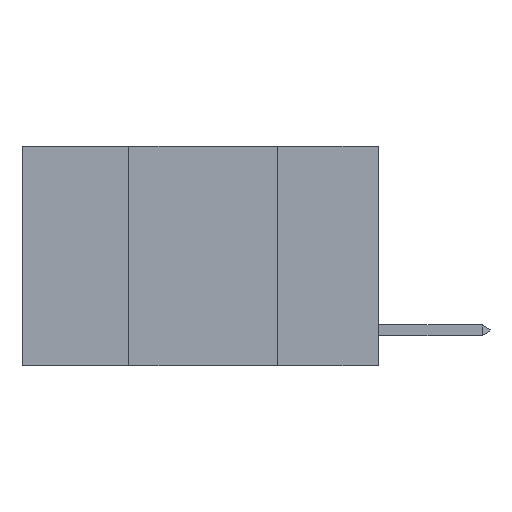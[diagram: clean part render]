
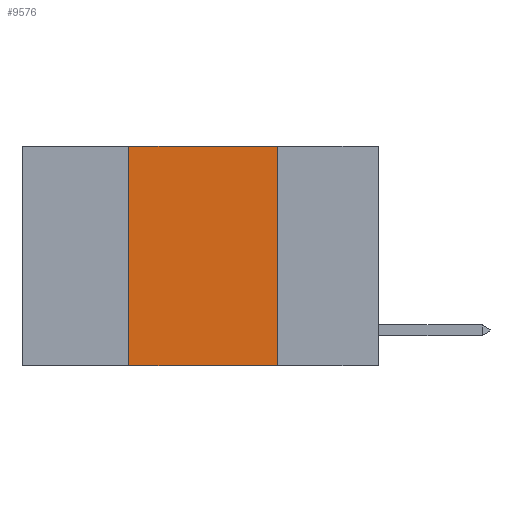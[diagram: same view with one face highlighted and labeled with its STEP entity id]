
A CAD part, left-side view. The second image highlights one B-rep face of the part: STEP entity #9576.
In plain terms, the highlighted planar face has unit normal (-1, 0, 0).
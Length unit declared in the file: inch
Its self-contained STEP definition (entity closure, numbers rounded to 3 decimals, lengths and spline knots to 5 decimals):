
#355 = VERTEX_POINT ( 'NONE', #8555 ) ;
#1116 = EDGE_CURVE ( 'NONE', #13549, #15274, #14706, .T. ) ;
#1256 = VECTOR ( 'NONE', #15183, 39.37008 ) ;
#1511 = CARTESIAN_POINT ( 'NONE',  ( 0., 0.6, 0. ) ) ;
#2590 = CARTESIAN_POINT ( 'NONE',  ( 0., 0.42, -0.37 ) ) ;
#3362 = ORIENTED_EDGE ( 'NONE', *, *, #14846, .T. ) ;
#4277 = PLANE ( 'NONE',  #7768 ) ;
#4465 = DIRECTION ( 'NONE',  ( 0., 0., -1. ) ) ;
#5555 = FACE_OUTER_BOUND ( 'NONE', #8623, .T. ) ;
#7768 = AXIS2_PLACEMENT_3D ( 'NONE', #18948, #8563, #4465 ) ;
#8332 = EDGE_CURVE ( 'NONE', #15429, #355, #17656, .T. ) ;
#8555 = CARTESIAN_POINT ( 'NONE',  ( 0., 0.42, 0. ) ) ;
#8563 = DIRECTION ( 'NONE',  ( 1., 0., 0. ) ) ;
#8623 = EDGE_LOOP ( 'NONE', ( #14347, #12231, #17965, #3362 ) ) ;
#8728 = CARTESIAN_POINT ( 'NONE',  ( 0., 0.17, 0. ) ) ;
#8741 = DIRECTION ( 'NONE',  ( 0., 0., 1. ) ) ;
#8814 = DIRECTION ( 'NONE',  ( 0., 0., -1. ) ) ;
#9192 = LINE ( 'NONE', #19212, #1256 ) ;
#9576 = ADVANCED_FACE ( 'NONE', ( #5555 ), #4277, .F. ) ;
#11822 = VECTOR ( 'NONE', #8814, 39.37008 ) ;
#12027 = DIRECTION ( 'NONE',  ( 0., -1., 0. ) ) ;
#12231 = ORIENTED_EDGE ( 'NONE', *, *, #13913, .F. ) ;
#13229 = LINE ( 'NONE', #1511, #17249 ) ;
#13549 = VERTEX_POINT ( 'NONE', #8728 ) ;
#13913 = EDGE_CURVE ( 'NONE', #355, #13549, #13229, .T. ) ;
#14347 = ORIENTED_EDGE ( 'NONE', *, *, #1116, .F. ) ;
#14706 = LINE ( 'NONE', #16447, #11822 ) ;
#14846 = EDGE_CURVE ( 'NONE', #15429, #15274, #9192, .T. ) ;
#15183 = DIRECTION ( 'NONE',  ( 0., -1., 0. ) ) ;
#15274 = VERTEX_POINT ( 'NONE', #17601 ) ;
#15429 = VERTEX_POINT ( 'NONE', #2590 ) ;
#16447 = CARTESIAN_POINT ( 'NONE',  ( 0., 0.17, 0. ) ) ;
#17249 = VECTOR ( 'NONE', #12027, 39.37008 ) ;
#17601 = CARTESIAN_POINT ( 'NONE',  ( 0., 0.17, -0.37 ) ) ;
#17656 = LINE ( 'NONE', #19035, #18620 ) ;
#17965 = ORIENTED_EDGE ( 'NONE', *, *, #8332, .F. ) ;
#18620 = VECTOR ( 'NONE', #8741, 39.37008 ) ;
#18948 = CARTESIAN_POINT ( 'NONE',  ( 0., 0.6, 0. ) ) ;
#19035 = CARTESIAN_POINT ( 'NONE',  ( 0., 0.42, 0. ) ) ;
#19212 = CARTESIAN_POINT ( 'NONE',  ( 0., 0.6, -0.37 ) ) ;
